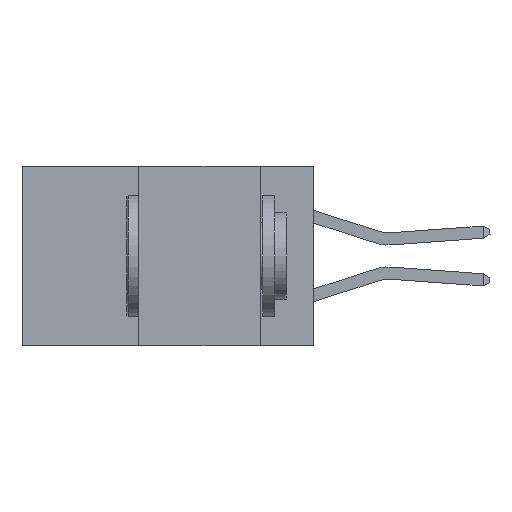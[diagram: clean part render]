
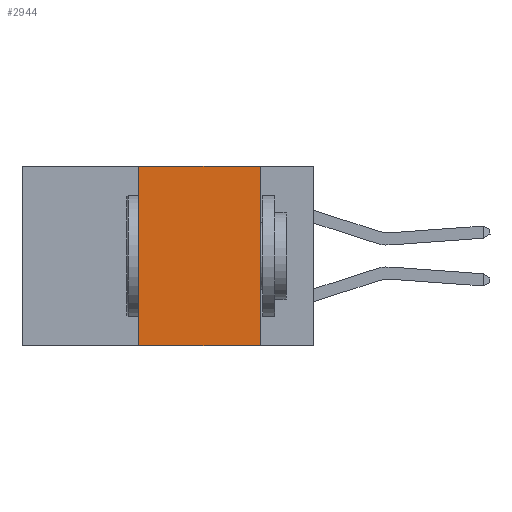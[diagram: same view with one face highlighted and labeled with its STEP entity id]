
A CAD part, left-side view. The second image highlights one B-rep face of the part: STEP entity #2944.
In plain terms, the highlighted planar face has unit normal (-1, 0, 0).
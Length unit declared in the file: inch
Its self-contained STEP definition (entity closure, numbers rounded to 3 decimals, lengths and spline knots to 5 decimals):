
#131 = EDGE_CURVE ( 'NONE', #2608, #13479, #10275, .T. ) ;
#914 = CARTESIAN_POINT ( 'NONE',  ( 0., 0.11, -0.37 ) ) ;
#1788 = ORIENTED_EDGE ( 'NONE', *, *, #5679, .F. ) ;
#2315 = VECTOR ( 'NONE', #2672, 39.37008 ) ;
#2608 = VERTEX_POINT ( 'NONE', #4299 ) ;
#2672 = DIRECTION ( 'NONE',  ( 0., 0., -1. ) ) ;
#2896 = CARTESIAN_POINT ( 'NONE',  ( 0., 0.11, 0. ) ) ;
#2944 = ADVANCED_FACE ( 'NONE', ( #3597 ), #12862, .F. ) ;
#3228 = VECTOR ( 'NONE', #10793, 39.37008 ) ;
#3597 = FACE_OUTER_BOUND ( 'NONE', #13267, .T. ) ;
#4046 = VECTOR ( 'NONE', #7341, 39.37008 ) ;
#4073 = DIRECTION ( 'NONE',  ( 0., 0., 1. ) ) ;
#4196 = EDGE_CURVE ( 'NONE', #11948, #10463, #5596, .T. ) ;
#4299 = CARTESIAN_POINT ( 'NONE',  ( 0., 0.36, 0. ) ) ;
#4376 = CARTESIAN_POINT ( 'NONE',  ( 0., 0.11, 0. ) ) ;
#5398 = LINE ( 'NONE', #2896, #2315 ) ;
#5479 = VECTOR ( 'NONE', #4073, 39.37008 ) ;
#5596 = LINE ( 'NONE', #10640, #3228 ) ;
#5679 = EDGE_CURVE ( 'NONE', #13479, #10463, #5398, .T. ) ;
#5968 = ORIENTED_EDGE ( 'NONE', *, *, #9579, .F. ) ;
#6679 = ORIENTED_EDGE ( 'NONE', *, *, #4196, .T. ) ;
#7341 = DIRECTION ( 'NONE',  ( 0., -1., 0. ) ) ;
#8395 = AXIS2_PLACEMENT_3D ( 'NONE', #13203, #12600, #12553 ) ;
#8548 = ORIENTED_EDGE ( 'NONE', *, *, #131, .F. ) ;
#8804 = CARTESIAN_POINT ( 'NONE',  ( 0., 0.6, 0. ) ) ;
#9395 = CARTESIAN_POINT ( 'NONE',  ( 0., 0.36, -0.37 ) ) ;
#9579 = EDGE_CURVE ( 'NONE', #11948, #2608, #14022, .T. ) ;
#10275 = LINE ( 'NONE', #8804, #4046 ) ;
#10463 = VERTEX_POINT ( 'NONE', #914 ) ;
#10640 = CARTESIAN_POINT ( 'NONE',  ( 0., 0.6, -0.37 ) ) ;
#10793 = DIRECTION ( 'NONE',  ( 0., -1., 0. ) ) ;
#11948 = VERTEX_POINT ( 'NONE', #9395 ) ;
#12553 = DIRECTION ( 'NONE',  ( 0., 0., -1. ) ) ;
#12600 = DIRECTION ( 'NONE',  ( 1., 0., 0. ) ) ;
#12862 = PLANE ( 'NONE',  #8395 ) ;
#13203 = CARTESIAN_POINT ( 'NONE',  ( 0., 0.6, 0. ) ) ;
#13267 = EDGE_LOOP ( 'NONE', ( #1788, #8548, #5968, #6679 ) ) ;
#13479 = VERTEX_POINT ( 'NONE', #4376 ) ;
#13791 = CARTESIAN_POINT ( 'NONE',  ( 0., 0.36, 0. ) ) ;
#14022 = LINE ( 'NONE', #13791, #5479 ) ;
